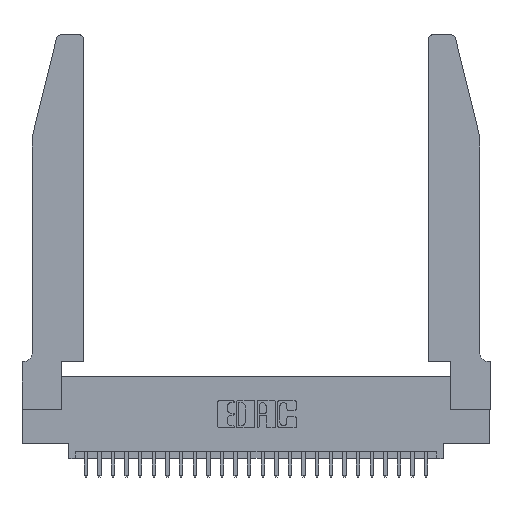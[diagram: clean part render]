
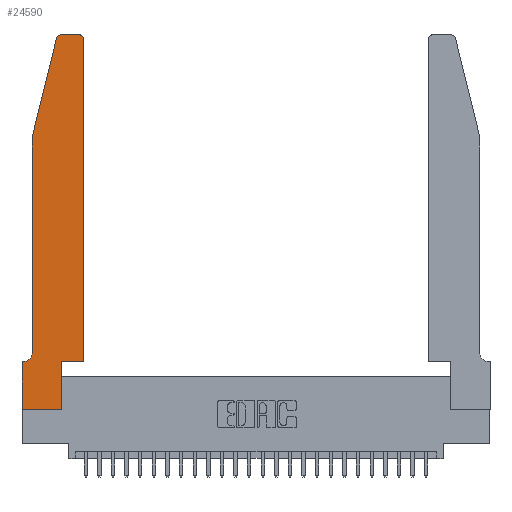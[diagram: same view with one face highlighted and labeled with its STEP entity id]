
A CAD part, top view. The second image highlights one B-rep face of the part: STEP entity #24590.
In plain terms, the highlighted planar face has unit normal (0, 0, 1).
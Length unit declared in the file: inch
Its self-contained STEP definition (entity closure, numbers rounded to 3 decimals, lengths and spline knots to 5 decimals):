
#161 = DIRECTION ( 'NONE',  ( -1., 0., 0. ) ) ;
#188 = CARTESIAN_POINT ( 'NONE',  ( 0.0755, 2., 0.37 ) ) ;
#275 = VERTEX_POINT ( 'NONE', #18668 ) ;
#957 = CARTESIAN_POINT ( 'NONE',  ( 0.0755, 2., 0.37 ) ) ;
#1916 = CIRCLE ( 'NONE', #5265, 0.03 ) ;
#2116 = VECTOR ( 'NONE', #161, 39.37008 ) ;
#2120 = AXIS2_PLACEMENT_3D ( 'NONE', #24325, #11426, #9591 ) ;
#2193 = CARTESIAN_POINT ( 'NONE',  ( 0.4505, 0.35, 0.37 ) ) ;
#2306 = LINE ( 'NONE', #16005, #12950 ) ;
#2480 = CARTESIAN_POINT ( 'NONE',  ( 0.0755, 0.35, 0.37 ) ) ;
#2540 = ORIENTED_EDGE ( 'NONE', *, *, #12885, .T. ) ;
#3148 = EDGE_CURVE ( 'NONE', #27210, #10323, #25994, .T. ) ;
#3303 = DIRECTION ( 'NONE',  ( 0., 0., -1. ) ) ;
#3882 = VERTEX_POINT ( 'NONE', #9056 ) ;
#3997 = PLANE ( 'NONE',  #20222 ) ;
#4204 = CIRCLE ( 'NONE', #11884, 0.07 ) ;
#4209 = DIRECTION ( 'NONE',  ( -0.239, -0.971, 0. ) ) ;
#4571 = CARTESIAN_POINT ( 'NONE',  ( 0.2865, 0., 0.37 ) ) ;
#4898 = CARTESIAN_POINT ( 'NONE',  ( 0.4505, 0.35, 0.37 ) ) ;
#5244 = CARTESIAN_POINT ( 'NONE',  ( 0.4505, 2.72, 0.37 ) ) ;
#5265 = AXIS2_PLACEMENT_3D ( 'NONE', #8585, #23509, #23422 ) ;
#5362 = ORIENTED_EDGE ( 'NONE', *, *, #9157, .T. ) ;
#6209 = LINE ( 'NONE', #957, #13509 ) ;
#6350 = DIRECTION ( 'NONE',  ( 0., 1., 0. ) ) ;
#6605 = VERTEX_POINT ( 'NONE', #10115 ) ;
#7567 = DIRECTION ( 'NONE',  ( -1., 0., 0. ) ) ;
#7621 = EDGE_CURVE ( 'NONE', #275, #6605, #4204, .T. ) ;
#7691 = VERTEX_POINT ( 'NONE', #16550 ) ;
#7825 = EDGE_CURVE ( 'NONE', #17563, #12683, #1916, .T. ) ;
#8282 = DIRECTION ( 'NONE',  ( 0., 0., 1. ) ) ;
#8466 = CARTESIAN_POINT ( 'NONE',  ( 0., 0.35, 0.37 ) ) ;
#8585 = CARTESIAN_POINT ( 'NONE',  ( 0.4205, 2.72, 0.37 ) ) ;
#8771 = CARTESIAN_POINT ( 'NONE',  ( 0.4505, 0.35, 0.37 ) ) ;
#9047 = VECTOR ( 'NONE', #23842, 39.37008 ) ;
#9056 = CARTESIAN_POINT ( 'NONE',  ( 0.2865, 0.35, 0.37 ) ) ;
#9157 = EDGE_CURVE ( 'NONE', #26511, #7691, #17762, .T. ) ;
#9591 = DIRECTION ( 'NONE',  ( 1., 0., 0. ) ) ;
#10115 = CARTESIAN_POINT ( 'NONE',  ( 0.0055, 0.35, 0.37 ) ) ;
#10323 = VERTEX_POINT ( 'NONE', #4571 ) ;
#10330 = EDGE_LOOP ( 'NONE', ( #2540, #5362, #19266, #22414, #14400, #13390, #27005, #16063, #22376, #17006, #12252, #18827 ) ) ;
#10608 = CARTESIAN_POINT ( 'NONE',  ( 0.284, 2.75, 0.37 ) ) ;
#10681 = DIRECTION ( 'NONE',  ( 1., 0., 0. ) ) ;
#10948 = CARTESIAN_POINT ( 'NONE',  ( 0., 0.35, 0.37 ) ) ;
#11426 = DIRECTION ( 'NONE',  ( 0., 0., 1. ) ) ;
#11439 = DIRECTION ( 'NONE',  ( 1., 0., 0. ) ) ;
#11884 = AXIS2_PLACEMENT_3D ( 'NONE', #15999, #3303, #7567 ) ;
#12108 = EDGE_CURVE ( 'NONE', #21998, #17563, #15979, .T. ) ;
#12252 = ORIENTED_EDGE ( 'NONE', *, *, #12108, .T. ) ;
#12683 = VERTEX_POINT ( 'NONE', #23541 ) ;
#12792 = CARTESIAN_POINT ( 'NONE',  ( 0.0755, 2., 0.37 ) ) ;
#12885 = EDGE_CURVE ( 'NONE', #12683, #26511, #2306, .T. ) ;
#12950 = VECTOR ( 'NONE', #26771, 39.37008 ) ;
#13389 = EDGE_CURVE ( 'NONE', #3882, #21998, #18926, .T. ) ;
#13390 = ORIENTED_EDGE ( 'NONE', *, *, #21336, .T. ) ;
#13509 = VECTOR ( 'NONE', #13678, 39.37008 ) ;
#13554 = CARTESIAN_POINT ( 'NONE',  ( 0., 0., 0.37 ) ) ;
#13678 = DIRECTION ( 'NONE',  ( 0., -1., 0. ) ) ;
#13801 = DIRECTION ( 'NONE',  ( 1., 0., 0. ) ) ;
#14400 = ORIENTED_EDGE ( 'NONE', *, *, #7621, .T. ) ;
#14462 = VECTOR ( 'NONE', #13801, 39.37008 ) ;
#14766 = VECTOR ( 'NONE', #6350, 39.37008 ) ;
#14914 = VECTOR ( 'NONE', #11439, 39.37008 ) ;
#15979 = LINE ( 'NONE', #4898, #25273 ) ;
#15999 = CARTESIAN_POINT ( 'NONE',  ( 0.0055, 0.42, 0.37 ) ) ;
#16005 = CARTESIAN_POINT ( 'NONE',  ( 0.2605, 2.75, 0.37 ) ) ;
#16063 = ORIENTED_EDGE ( 'NONE', *, *, #3148, .T. ) ;
#16550 = CARTESIAN_POINT ( 'NONE',  ( 0.25487, 2.72718, 0.37 ) ) ;
#17006 = ORIENTED_EDGE ( 'NONE', *, *, #13389, .T. ) ;
#17563 = VERTEX_POINT ( 'NONE', #5244 ) ;
#17762 = CIRCLE ( 'NONE', #2120, 0.03 ) ;
#18386 = LINE ( 'NONE', #2480, #2116 ) ;
#18668 = CARTESIAN_POINT ( 'NONE',  ( 0.0755, 0.42, 0.37 ) ) ;
#18827 = ORIENTED_EDGE ( 'NONE', *, *, #7825, .T. ) ;
#18926 = LINE ( 'NONE', #8771, #14914 ) ;
#18980 = VECTOR ( 'NONE', #4209, 39.37008 ) ;
#19266 = ORIENTED_EDGE ( 'NONE', *, *, #21820, .T. ) ;
#19514 = DIRECTION ( 'NONE',  ( 0., 1., 0. ) ) ;
#20222 = AXIS2_PLACEMENT_3D ( 'NONE', #8466, #8282, #10681 ) ;
#20512 = CARTESIAN_POINT ( 'NONE',  ( 0.2865, 0.35, 0.37 ) ) ;
#21336 = EDGE_CURVE ( 'NONE', #6605, #22502, #18386, .T. ) ;
#21340 = LINE ( 'NONE', #13554, #9047 ) ;
#21472 = FACE_OUTER_BOUND ( 'NONE', #10330, .T. ) ;
#21820 = EDGE_CURVE ( 'NONE', #7691, #27029, #24588, .T. ) ;
#21998 = VERTEX_POINT ( 'NONE', #2193 ) ;
#22376 = ORIENTED_EDGE ( 'NONE', *, *, #25684, .T. ) ;
#22414 = ORIENTED_EDGE ( 'NONE', *, *, #24412, .T. ) ;
#22502 = VERTEX_POINT ( 'NONE', #10948 ) ;
#23422 = DIRECTION ( 'NONE',  ( 1., 0., 0. ) ) ;
#23509 = DIRECTION ( 'NONE',  ( 0., 0., 1. ) ) ;
#23541 = CARTESIAN_POINT ( 'NONE',  ( 0.4205, 2.75, 0.37 ) ) ;
#23842 = DIRECTION ( 'NONE',  ( 0., -1., 0. ) ) ;
#23898 = CARTESIAN_POINT ( 'NONE',  ( 0., 0., 0.37 ) ) ;
#24325 = CARTESIAN_POINT ( 'NONE',  ( 0.284, 2.72, 0.37 ) ) ;
#24412 = EDGE_CURVE ( 'NONE', #27029, #275, #6209, .T. ) ;
#24588 = LINE ( 'NONE', #12792, #18980 ) ;
#24590 = ADVANCED_FACE ( 'NONE', ( #21472 ), #3997, .T. ) ;
#24693 = LINE ( 'NONE', #20512, #14766 ) ;
#25273 = VECTOR ( 'NONE', #19514, 39.37008 ) ;
#25684 = EDGE_CURVE ( 'NONE', #10323, #3882, #24693, .T. ) ;
#25994 = LINE ( 'NONE', #23898, #14462 ) ;
#26431 = CARTESIAN_POINT ( 'NONE',  ( 0., 0., 0.37 ) ) ;
#26511 = VERTEX_POINT ( 'NONE', #10608 ) ;
#26586 = EDGE_CURVE ( 'NONE', #22502, #27210, #21340, .T. ) ;
#26771 = DIRECTION ( 'NONE',  ( -1., 0., 0. ) ) ;
#27005 = ORIENTED_EDGE ( 'NONE', *, *, #26586, .T. ) ;
#27029 = VERTEX_POINT ( 'NONE', #188 ) ;
#27210 = VERTEX_POINT ( 'NONE', #26431 ) ;
